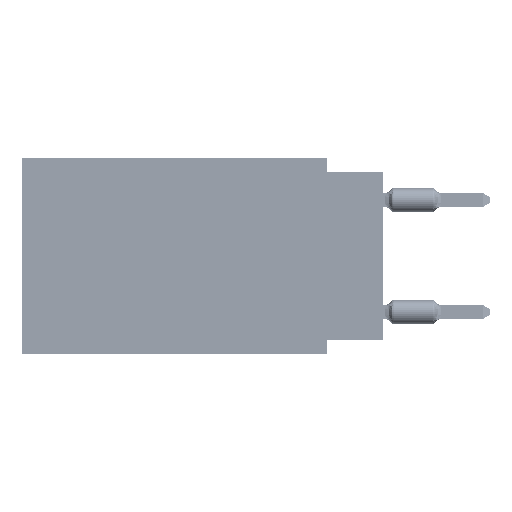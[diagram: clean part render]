
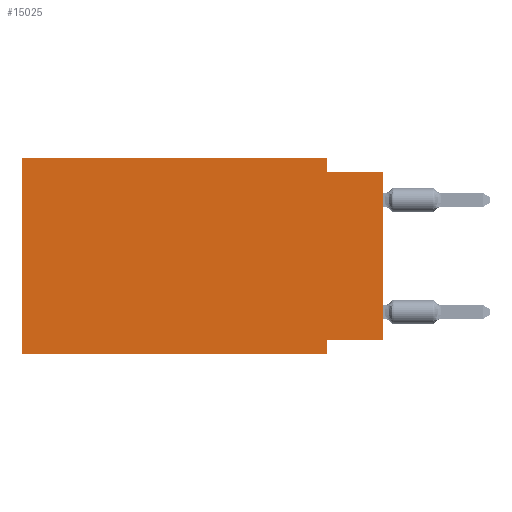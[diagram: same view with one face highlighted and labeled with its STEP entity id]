
A CAD part, left-side view. The second image highlights one B-rep face of the part: STEP entity #15025.
In plain terms, the highlighted planar face has unit normal (-1, 0, 0).
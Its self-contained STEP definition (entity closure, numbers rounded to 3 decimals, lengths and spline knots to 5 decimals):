
#2220 = EDGE_LOOP ( 'NONE', ( #76655, #109364, #69134, #7982, #20264, #37582, #6858, #70710 ) ) ;
#2937 = VECTOR ( 'NONE', #83494, 39.37008 ) ;
#4666 = VECTOR ( 'NONE', #25956, 39.37008 ) ;
#6858 = ORIENTED_EDGE ( 'NONE', *, *, #15615, .F. ) ;
#7982 = ORIENTED_EDGE ( 'NONE', *, *, #31368, .F. ) ;
#8346 = EDGE_CURVE ( 'NONE', #101449, #113886, #78978, .T. ) ;
#8546 = VECTOR ( 'NONE', #15099, 39.37008 ) ;
#9005 = CARTESIAN_POINT ( 'NONE',  ( 0., 0.645, -0.35 ) ) ;
#11378 = LINE ( 'NONE', #75262, #2937 ) ;
#13215 = VERTEX_POINT ( 'NONE', #111431 ) ;
#14669 = DIRECTION ( 'NONE',  ( 0., 0., -1. ) ) ;
#15025 = ADVANCED_FACE ( 'NONE', ( #77411 ), #83902, .F. ) ;
#15099 = DIRECTION ( 'NONE',  ( 0., 0., -1. ) ) ;
#15615 = EDGE_CURVE ( 'NONE', #34461, #57167, #50902, .T. ) ;
#16166 = VECTOR ( 'NONE', #111363, 39.37008 ) ;
#20264 = ORIENTED_EDGE ( 'NONE', *, *, #84582, .F. ) ;
#25956 = DIRECTION ( 'NONE',  ( 0., 0., 1. ) ) ;
#27692 = LINE ( 'NONE', #99182, #4666 ) ;
#27882 = CARTESIAN_POINT ( 'NONE',  ( 0., 0., -0.025 ) ) ;
#30347 = EDGE_CURVE ( 'NONE', #13215, #39837, #27692, .T. ) ;
#31368 = EDGE_CURVE ( 'NONE', #93570, #101449, #45664, .T. ) ;
#33684 = LINE ( 'NONE', #9005, #89544 ) ;
#34461 = VERTEX_POINT ( 'NONE', #87309 ) ;
#35059 = EDGE_CURVE ( 'NONE', #76337, #57167, #33684, .T. ) ;
#35594 = DIRECTION ( 'NONE',  ( 0., 0., -1. ) ) ;
#36776 = CARTESIAN_POINT ( 'NONE',  ( 0., 0.1, 0. ) ) ;
#37582 = ORIENTED_EDGE ( 'NONE', *, *, #35059, .T. ) ;
#37804 = VECTOR ( 'NONE', #98229, 39.37008 ) ;
#39064 = CARTESIAN_POINT ( 'NONE',  ( 0., 0.1, -0.35 ) ) ;
#39837 = VERTEX_POINT ( 'NONE', #83863 ) ;
#45664 = LINE ( 'NONE', #91940, #60858 ) ;
#49813 = CARTESIAN_POINT ( 'NONE',  ( 0., 0., -0.325 ) ) ;
#50902 = LINE ( 'NONE', #95416, #8546 ) ;
#57167 = VERTEX_POINT ( 'NONE', #39064 ) ;
#57692 = CARTESIAN_POINT ( 'NONE',  ( 0., 0.1, 0. ) ) ;
#60858 = VECTOR ( 'NONE', #91373, 39.37008 ) ;
#63264 = EDGE_CURVE ( 'NONE', #113886, #39837, #97649, .T. ) ;
#69134 = ORIENTED_EDGE ( 'NONE', *, *, #8346, .F. ) ;
#69428 = DIRECTION ( 'NONE',  ( 0., -1., 0. ) ) ;
#70710 = ORIENTED_EDGE ( 'NONE', *, *, #104869, .F. ) ;
#75262 = CARTESIAN_POINT ( 'NONE',  ( 0., 0.645, 0. ) ) ;
#76337 = VERTEX_POINT ( 'NONE', #113389 ) ;
#76655 = ORIENTED_EDGE ( 'NONE', *, *, #30347, .T. ) ;
#77411 = FACE_OUTER_BOUND ( 'NONE', #2220, .T. ) ;
#78978 = LINE ( 'NONE', #36776, #80526 ) ;
#80526 = VECTOR ( 'NONE', #35594, 39.37008 ) ;
#83494 = DIRECTION ( 'NONE',  ( 0., 0., 1. ) ) ;
#83863 = CARTESIAN_POINT ( 'NONE',  ( 0., 0., -0.025 ) ) ;
#83902 = PLANE ( 'NONE',  #100212 ) ;
#84582 = EDGE_CURVE ( 'NONE', #76337, #93570, #11378, .T. ) ;
#87309 = CARTESIAN_POINT ( 'NONE',  ( 0., 0.1, -0.325 ) ) ;
#89544 = VECTOR ( 'NONE', #69428, 39.37008 ) ;
#91373 = DIRECTION ( 'NONE',  ( 0., -1., 0. ) ) ;
#91940 = CARTESIAN_POINT ( 'NONE',  ( 0., 0.645, 0. ) ) ;
#93480 = CARTESIAN_POINT ( 'NONE',  ( 0., 0.645, 0. ) ) ;
#93570 = VERTEX_POINT ( 'NONE', #93480 ) ;
#93846 = CARTESIAN_POINT ( 'NONE',  ( 0., 0.1, -0.025 ) ) ;
#95416 = CARTESIAN_POINT ( 'NONE',  ( 0., 0.1, -0.35 ) ) ;
#97649 = LINE ( 'NONE', #27882, #37804 ) ;
#98229 = DIRECTION ( 'NONE',  ( 0., -1., 0. ) ) ;
#99182 = CARTESIAN_POINT ( 'NONE',  ( 0., 0., 0. ) ) ;
#100212 = AXIS2_PLACEMENT_3D ( 'NONE', #104366, #103793, #14669 ) ;
#101449 = VERTEX_POINT ( 'NONE', #57692 ) ;
#103793 = DIRECTION ( 'NONE',  ( 1., 0., 0. ) ) ;
#104366 = CARTESIAN_POINT ( 'NONE',  ( 0., 0.645, 0. ) ) ;
#104869 = EDGE_CURVE ( 'NONE', #13215, #34461, #112535, .T. ) ;
#109364 = ORIENTED_EDGE ( 'NONE', *, *, #63264, .F. ) ;
#111363 = DIRECTION ( 'NONE',  ( 0., 1., 0. ) ) ;
#111431 = CARTESIAN_POINT ( 'NONE',  ( 0., 0., -0.325 ) ) ;
#112535 = LINE ( 'NONE', #49813, #16166 ) ;
#113389 = CARTESIAN_POINT ( 'NONE',  ( 0., 0.645, -0.35 ) ) ;
#113886 = VERTEX_POINT ( 'NONE', #93846 ) ;
